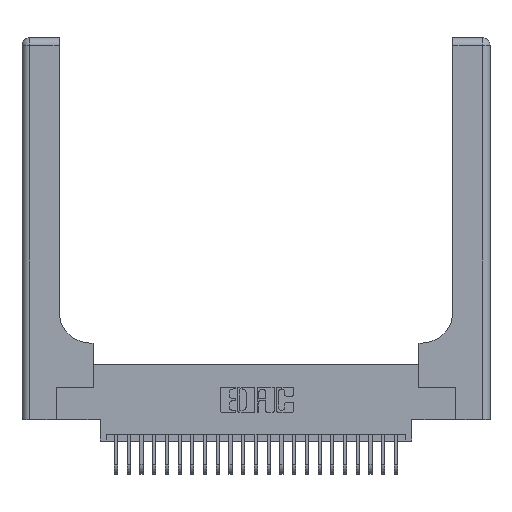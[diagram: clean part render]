
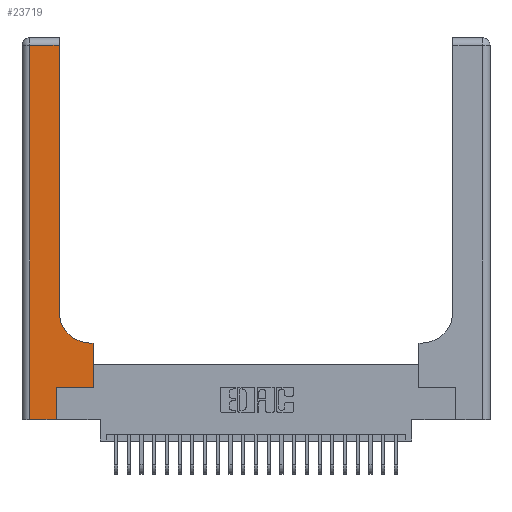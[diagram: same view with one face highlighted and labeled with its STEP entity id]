
A CAD part, top view. The second image highlights one B-rep face of the part: STEP entity #23719.
In plain terms, the highlighted planar face has unit normal (0, 0, 1).
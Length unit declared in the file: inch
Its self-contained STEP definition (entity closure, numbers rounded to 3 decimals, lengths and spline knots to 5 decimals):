
#27 = VECTOR ( 'NONE', #3539, 39.37008 ) ;
#206 = LINE ( 'NONE', #24567, #10053 ) ;
#773 = DIRECTION ( 'NONE',  ( 0., 1., 0. ) ) ;
#1231 = CARTESIAN_POINT ( 'NONE',  ( 0.269, 0., 0.37 ) ) ;
#2077 = EDGE_CURVE ( 'NONE', #23883, #23960, #19896, .T. ) ;
#2097 = ORIENTED_EDGE ( 'NONE', *, *, #10958, .T. ) ;
#2763 = CARTESIAN_POINT ( 'NONE',  ( 0.269, 0.25, 0.37 ) ) ;
#3162 = VECTOR ( 'NONE', #24788, 39.37008 ) ;
#3539 = DIRECTION ( 'NONE',  ( 1., 0., 0. ) ) ;
#3663 = CARTESIAN_POINT ( 'NONE',  ( 0.5585, 0.25, 0.37 ) ) ;
#3814 = CARTESIAN_POINT ( 'NONE',  ( 0.06, 0., 0.37 ) ) ;
#3865 = ORIENTED_EDGE ( 'NONE', *, *, #6693, .T. ) ;
#4726 = VERTEX_POINT ( 'NONE', #3814 ) ;
#5305 = EDGE_LOOP ( 'NONE', ( #18488, #14170, #17687, #3865, #23928, #2097, #16893, #19879, #19414 ) ) ;
#5371 = EDGE_CURVE ( 'NONE', #17533, #19682, #17033, .T. ) ;
#5478 = CARTESIAN_POINT ( 'NONE',  ( 0.269, 0.25, 0.37 ) ) ;
#6196 = EDGE_CURVE ( 'NONE', #15397, #7190, #24509, .T. ) ;
#6292 = VERTEX_POINT ( 'NONE', #3663 ) ;
#6539 = DIRECTION ( 'NONE',  ( 0., 0., -1. ) ) ;
#6693 = EDGE_CURVE ( 'NONE', #4726, #15397, #19377, .T. ) ;
#7190 = VERTEX_POINT ( 'NONE', #2763 ) ;
#7802 = EDGE_CURVE ( 'NONE', #6292, #17533, #13849, .T. ) ;
#7847 = FACE_OUTER_BOUND ( 'NONE', #5305, .T. ) ;
#8686 = AXIS2_PLACEMENT_3D ( 'NONE', #21226, #9527, #23134 ) ;
#8800 = EDGE_CURVE ( 'NONE', #23960, #12720, #19785, .T. ) ;
#9327 = CIRCLE ( 'NONE', #8686, 0.25 ) ;
#9527 = DIRECTION ( 'NONE',  ( 0., 0., -1. ) ) ;
#9549 = CARTESIAN_POINT ( 'NONE',  ( 0.06, 2.94, 0.37 ) ) ;
#10053 = VECTOR ( 'NONE', #13018, 39.37008 ) ;
#10883 = DIRECTION ( 'NONE',  ( 1., 0., 0. ) ) ;
#10958 = EDGE_CURVE ( 'NONE', #7190, #6292, #15712, .T. ) ;
#11171 = CARTESIAN_POINT ( 'NONE',  ( 0.2915, 2.94, 0.37 ) ) ;
#12051 = CARTESIAN_POINT ( 'NONE',  ( 0.2915, 3., 0.37 ) ) ;
#12589 = CARTESIAN_POINT ( 'NONE',  ( 0.2915, 0.6, 0.37 ) ) ;
#12720 = VERTEX_POINT ( 'NONE', #9549 ) ;
#13016 = VECTOR ( 'NONE', #10883, 39.37008 ) ;
#13018 = DIRECTION ( 'NONE',  ( 0., -1., 0. ) ) ;
#13245 = CARTESIAN_POINT ( 'NONE',  ( 0.269, 0., 0.37 ) ) ;
#13849 = LINE ( 'NONE', #14547, #18423 ) ;
#14116 = AXIS2_PLACEMENT_3D ( 'NONE', #18279, #6539, #20229 ) ;
#14170 = ORIENTED_EDGE ( 'NONE', *, *, #8800, .T. ) ;
#14267 = EDGE_CURVE ( 'NONE', #12720, #4726, #206, .T. ) ;
#14547 = CARTESIAN_POINT ( 'NONE',  ( 0.5585, 0.25, 0.37 ) ) ;
#14607 = CARTESIAN_POINT ( 'NONE',  ( 0.5585, 0.6, 0.37 ) ) ;
#14672 = DIRECTION ( 'NONE',  ( -1., 0., 0. ) ) ;
#15397 = VERTEX_POINT ( 'NONE', #1231 ) ;
#15712 = LINE ( 'NONE', #5478, #27 ) ;
#15808 = VECTOR ( 'NONE', #20424, 39.37008 ) ;
#16893 = ORIENTED_EDGE ( 'NONE', *, *, #7802, .T. ) ;
#17033 = LINE ( 'NONE', #12589, #15808 ) ;
#17533 = VERTEX_POINT ( 'NONE', #14607 ) ;
#17687 = ORIENTED_EDGE ( 'NONE', *, *, #14267, .T. ) ;
#17904 = CARTESIAN_POINT ( 'NONE',  ( 0.5415, 0.6, 0.37 ) ) ;
#18279 = CARTESIAN_POINT ( 'NONE',  ( 0., 3., 0.37 ) ) ;
#18423 = VECTOR ( 'NONE', #773, 39.37008 ) ;
#18488 = ORIENTED_EDGE ( 'NONE', *, *, #2077, .T. ) ;
#18502 = CARTESIAN_POINT ( 'NONE',  ( 0., 2.94, 0.37 ) ) ;
#18663 = CARTESIAN_POINT ( 'NONE',  ( 0., 0., 0.37 ) ) ;
#19271 = VECTOR ( 'NONE', #23645, 39.37008 ) ;
#19377 = LINE ( 'NONE', #18663, #13016 ) ;
#19414 = ORIENTED_EDGE ( 'NONE', *, *, #24778, .T. ) ;
#19682 = VERTEX_POINT ( 'NONE', #17904 ) ;
#19785 = LINE ( 'NONE', #18502, #22186 ) ;
#19879 = ORIENTED_EDGE ( 'NONE', *, *, #5371, .T. ) ;
#19896 = LINE ( 'NONE', #12051, #19271 ) ;
#20229 = DIRECTION ( 'NONE',  ( -1., 0., 0. ) ) ;
#20424 = DIRECTION ( 'NONE',  ( -1., 0., 0. ) ) ;
#21226 = CARTESIAN_POINT ( 'NONE',  ( 0.5415, 0.85, 0.37 ) ) ;
#22186 = VECTOR ( 'NONE', #14672, 39.37008 ) ;
#22552 = CARTESIAN_POINT ( 'NONE',  ( 0.2915, 0.85, 0.37 ) ) ;
#23134 = DIRECTION ( 'NONE',  ( 1., 0., 0. ) ) ;
#23645 = DIRECTION ( 'NONE',  ( 0., 1., 0. ) ) ;
#23719 = ADVANCED_FACE ( 'NONE', ( #7847 ), #23972, .F. ) ;
#23883 = VERTEX_POINT ( 'NONE', #22552 ) ;
#23928 = ORIENTED_EDGE ( 'NONE', *, *, #6196, .T. ) ;
#23960 = VERTEX_POINT ( 'NONE', #11171 ) ;
#23972 = PLANE ( 'NONE',  #14116 ) ;
#24509 = LINE ( 'NONE', #13245, #3162 ) ;
#24567 = CARTESIAN_POINT ( 'NONE',  ( 0.06, 3., 0.37 ) ) ;
#24778 = EDGE_CURVE ( 'NONE', #19682, #23883, #9327, .T. ) ;
#24788 = DIRECTION ( 'NONE',  ( 0., 1., 0. ) ) ;
